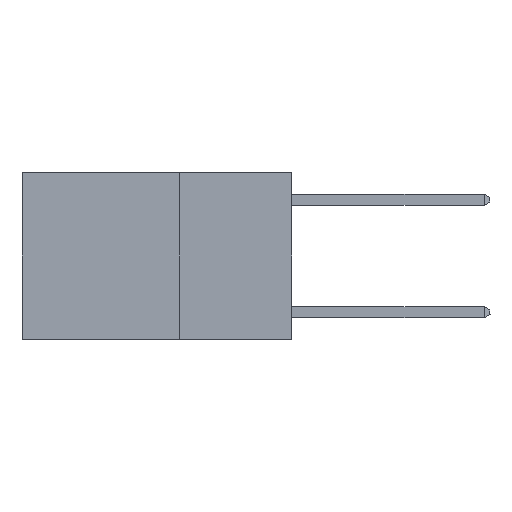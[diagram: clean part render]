
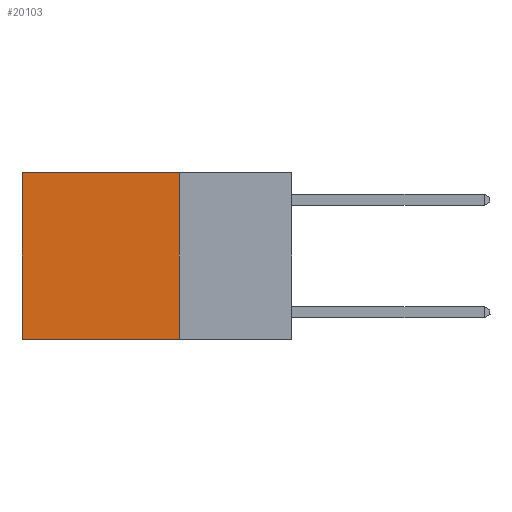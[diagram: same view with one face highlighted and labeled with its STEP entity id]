
A CAD part, left-side view. The second image highlights one B-rep face of the part: STEP entity #20103.
In plain terms, the highlighted planar face has unit normal (-1, 0, 0).
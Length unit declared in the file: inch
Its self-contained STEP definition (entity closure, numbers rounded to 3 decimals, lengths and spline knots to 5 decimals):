
#84 = EDGE_CURVE ( 'NONE', #17705, #1857, #20973, .T. ) ;
#362 = CARTESIAN_POINT ( 'NONE',  ( 0.2625, 0.25, 0. ) ) ;
#485 = EDGE_CURVE ( 'NONE', #4149, #10627, #10454, .T. ) ;
#831 = DIRECTION ( 'NONE',  ( 0., 1., 0. ) ) ;
#879 = PLANE ( 'NONE',  #22216 ) ;
#1531 = CARTESIAN_POINT ( 'NONE',  ( 0.2625, 0.6, -0.37 ) ) ;
#1857 = VERTEX_POINT ( 'NONE', #1531 ) ;
#3257 = ORIENTED_EDGE ( 'NONE', *, *, #84, .T. ) ;
#3927 = DIRECTION ( 'NONE',  ( 0., 0., -1. ) ) ;
#4149 = VERTEX_POINT ( 'NONE', #362 ) ;
#4556 = ORIENTED_EDGE ( 'NONE', *, *, #24033, .F. ) ;
#5538 = ORIENTED_EDGE ( 'NONE', *, *, #485, .F. ) ;
#7138 = FACE_OUTER_BOUND ( 'NONE', #22498, .T. ) ;
#9160 = DIRECTION ( 'NONE',  ( 0., 0., -1. ) ) ;
#10454 = LINE ( 'NONE', #18739, #21463 ) ;
#10592 = VECTOR ( 'NONE', #23187, 39.37008 ) ;
#10627 = VERTEX_POINT ( 'NONE', #14978 ) ;
#10644 = DIRECTION ( 'NONE',  ( 0., 0., -1. ) ) ;
#13109 = CARTESIAN_POINT ( 'NONE',  ( 0.2625, 0.25, -0.37 ) ) ;
#13219 = CARTESIAN_POINT ( 'NONE',  ( 0.2625, 0.25, 0. ) ) ;
#14978 = CARTESIAN_POINT ( 'NONE',  ( 0.2625, 0.25, -0.37 ) ) ;
#15595 = EDGE_CURVE ( 'NONE', #4149, #17705, #23563, .T. ) ;
#17705 = VERTEX_POINT ( 'NONE', #18411 ) ;
#18308 = VECTOR ( 'NONE', #831, 39.37008 ) ;
#18411 = CARTESIAN_POINT ( 'NONE',  ( 0.2625, 0.6, 0. ) ) ;
#18739 = CARTESIAN_POINT ( 'NONE',  ( 0.2625, 0.25, 0. ) ) ;
#18801 = CARTESIAN_POINT ( 'NONE',  ( 0.2625, 0.6, 0. ) ) ;
#19358 = DIRECTION ( 'NONE',  ( 1., 0., 0. ) ) ;
#20064 = ORIENTED_EDGE ( 'NONE', *, *, #15595, .T. ) ;
#20103 = ADVANCED_FACE ( 'NONE', ( #7138 ), #879, .F. ) ;
#20973 = LINE ( 'NONE', #18801, #22602 ) ;
#21114 = LINE ( 'NONE', #13109, #10592 ) ;
#21463 = VECTOR ( 'NONE', #3927, 39.37008 ) ;
#22216 = AXIS2_PLACEMENT_3D ( 'NONE', #23462, #19358, #9160 ) ;
#22498 = EDGE_LOOP ( 'NONE', ( #3257, #4556, #5538, #20064 ) ) ;
#22602 = VECTOR ( 'NONE', #10644, 39.37008 ) ;
#23187 = DIRECTION ( 'NONE',  ( 0., 1., 0. ) ) ;
#23462 = CARTESIAN_POINT ( 'NONE',  ( 0.2625, 0.25, 0. ) ) ;
#23563 = LINE ( 'NONE', #13219, #18308 ) ;
#24033 = EDGE_CURVE ( 'NONE', #10627, #1857, #21114, .T. ) ;
